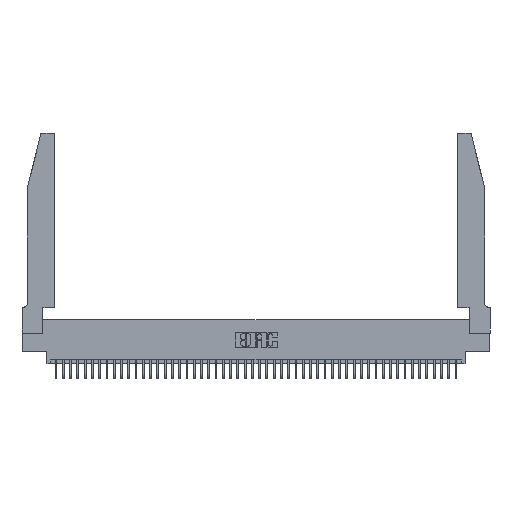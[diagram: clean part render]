
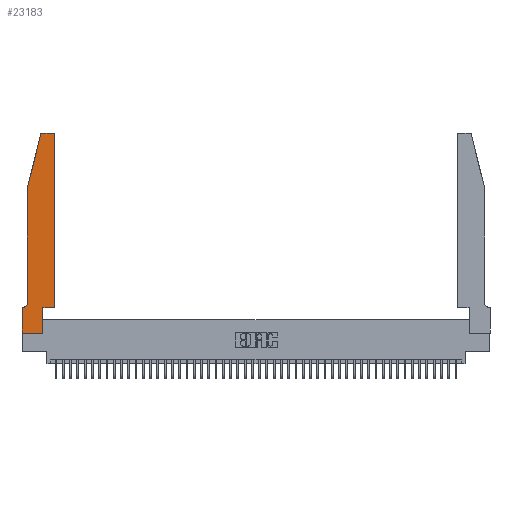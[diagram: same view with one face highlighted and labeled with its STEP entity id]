
A CAD part, top view. The second image highlights one B-rep face of the part: STEP entity #23183.
In plain terms, the highlighted planar face has unit normal (0, 0, 1).
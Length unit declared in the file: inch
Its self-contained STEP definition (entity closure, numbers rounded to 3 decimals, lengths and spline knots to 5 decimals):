
#257 = EDGE_CURVE ( 'NONE', #10455, #32081, #35449, .T. ) ;
#485 = VECTOR ( 'NONE', #39460, 39.37008 ) ;
#1752 = DIRECTION ( 'NONE',  ( 1., 0., 0. ) ) ;
#1906 = ORIENTED_EDGE ( 'NONE', *, *, #47987, .T. ) ;
#2184 = CARTESIAN_POINT ( 'NONE',  ( 0., 0.35, 0.37 ) ) ;
#2358 = DIRECTION ( 'NONE',  ( 1., 0., 0. ) ) ;
#2949 = CARTESIAN_POINT ( 'NONE',  ( 0.284, 2.72, 0.37 ) ) ;
#3360 = LINE ( 'NONE', #16788, #43288 ) ;
#3630 = CARTESIAN_POINT ( 'NONE',  ( 0.4205, 2.72, 0.37 ) ) ;
#4280 = VECTOR ( 'NONE', #7873, 39.37008 ) ;
#4769 = VERTEX_POINT ( 'NONE', #36016 ) ;
#4909 = AXIS2_PLACEMENT_3D ( 'NONE', #2184, #25086, #2358 ) ;
#5660 = CARTESIAN_POINT ( 'NONE',  ( 0.284, 2.75, 0.37 ) ) ;
#5737 = CARTESIAN_POINT ( 'NONE',  ( 0.4505, 0.35, 0.37 ) ) ;
#6211 = ORIENTED_EDGE ( 'NONE', *, *, #22383, .T. ) ;
#6527 = EDGE_CURVE ( 'NONE', #10375, #11061, #22239, .T. ) ;
#6867 = DIRECTION ( 'NONE',  ( 1., 0., 0. ) ) ;
#7563 = DIRECTION ( 'NONE',  ( 1., 0., 0. ) ) ;
#7873 = DIRECTION ( 'NONE',  ( 0., 1., 0. ) ) ;
#10061 = LINE ( 'NONE', #23931, #38669 ) ;
#10171 = LINE ( 'NONE', #46682, #19089 ) ;
#10375 = VERTEX_POINT ( 'NONE', #46897 ) ;
#10455 = VERTEX_POINT ( 'NONE', #28795 ) ;
#10740 = CARTESIAN_POINT ( 'NONE',  ( 0.4505, 0.35, 0.37 ) ) ;
#11061 = VERTEX_POINT ( 'NONE', #5660 ) ;
#11634 = ORIENTED_EDGE ( 'NONE', *, *, #18474, .T. ) ;
#11763 = CARTESIAN_POINT ( 'NONE',  ( 0.0055, 0.35, 0.37 ) ) ;
#12152 = DIRECTION ( 'NONE',  ( 0., 0., -1. ) ) ;
#12297 = ORIENTED_EDGE ( 'NONE', *, *, #15360, .T. ) ;
#14671 = VERTEX_POINT ( 'NONE', #47260 ) ;
#14941 = VERTEX_POINT ( 'NONE', #41276 ) ;
#15360 = EDGE_CURVE ( 'NONE', #37790, #4769, #41450, .T. ) ;
#15671 = VECTOR ( 'NONE', #40970, 39.37008 ) ;
#16411 = AXIS2_PLACEMENT_3D ( 'NONE', #34490, #12152, #38216 ) ;
#16788 = CARTESIAN_POINT ( 'NONE',  ( 0.0755, 2., 0.37 ) ) ;
#17345 = EDGE_CURVE ( 'NONE', #47071, #14671, #29085, .T. ) ;
#17365 = CARTESIAN_POINT ( 'NONE',  ( 0.2605, 2.75, 0.37 ) ) ;
#18474 = EDGE_CURVE ( 'NONE', #14671, #42699, #21819, .T. ) ;
#19089 = VECTOR ( 'NONE', #1752, 39.37008 ) ;
#20352 = CIRCLE ( 'NONE', #20672, 0.03 ) ;
#20645 = VECTOR ( 'NONE', #39708, 39.37008 ) ;
#20672 = AXIS2_PLACEMENT_3D ( 'NONE', #3630, #30081, #7563 ) ;
#21819 = LINE ( 'NONE', #35990, #20645 ) ;
#21844 = EDGE_CURVE ( 'NONE', #26323, #47071, #22605, .T. ) ;
#22239 = LINE ( 'NONE', #17365, #32104 ) ;
#22383 = EDGE_CURVE ( 'NONE', #42699, #10455, #10171, .T. ) ;
#22605 = CIRCLE ( 'NONE', #16411, 0.07 ) ;
#23183 = ADVANCED_FACE ( 'NONE', ( #42199 ), #32407, .T. ) ;
#23386 = ORIENTED_EDGE ( 'NONE', *, *, #31777, .T. ) ;
#23844 = CARTESIAN_POINT ( 'NONE',  ( 0.4505, 0.35, 0.37 ) ) ;
#23931 = CARTESIAN_POINT ( 'NONE',  ( 0.0755, 2., 0.37 ) ) ;
#24482 = ORIENTED_EDGE ( 'NONE', *, *, #30125, .T. ) ;
#25086 = DIRECTION ( 'NONE',  ( 0., 0., 1. ) ) ;
#25728 = ORIENTED_EDGE ( 'NONE', *, *, #27116, .T. ) ;
#25966 = VERTEX_POINT ( 'NONE', #30491 ) ;
#26323 = VERTEX_POINT ( 'NONE', #35918 ) ;
#27116 = EDGE_CURVE ( 'NONE', #4769, #10375, #20352, .T. ) ;
#27422 = ORIENTED_EDGE ( 'NONE', *, *, #43265, .T. ) ;
#27886 = DIRECTION ( 'NONE',  ( -0.239, -0.971, 0. ) ) ;
#28019 = ORIENTED_EDGE ( 'NONE', *, *, #17345, .T. ) ;
#28795 = CARTESIAN_POINT ( 'NONE',  ( 0.2865, 0., 0.37 ) ) ;
#29085 = LINE ( 'NONE', #48417, #15671 ) ;
#29406 = DIRECTION ( 'NONE',  ( 0., 0., 1. ) ) ;
#29792 = ORIENTED_EDGE ( 'NONE', *, *, #257, .T. ) ;
#30081 = DIRECTION ( 'NONE',  ( 0., 0., 1. ) ) ;
#30104 = CARTESIAN_POINT ( 'NONE',  ( 0.2865, 0.35, 0.37 ) ) ;
#30125 = EDGE_CURVE ( 'NONE', #25966, #26323, #10061, .T. ) ;
#30491 = CARTESIAN_POINT ( 'NONE',  ( 0.0755, 2., 0.37 ) ) ;
#30708 = LINE ( 'NONE', #5737, #485 ) ;
#31439 = DIRECTION ( 'NONE',  ( 0., -1., 0. ) ) ;
#31600 = VECTOR ( 'NONE', #40554, 39.37008 ) ;
#31777 = EDGE_CURVE ( 'NONE', #32081, #37790, #30708, .T. ) ;
#32081 = VERTEX_POINT ( 'NONE', #30104 ) ;
#32104 = VECTOR ( 'NONE', #43339, 39.37008 ) ;
#32407 = PLANE ( 'NONE',  #4909 ) ;
#34086 = CARTESIAN_POINT ( 'NONE',  ( 0.2865, 0.35, 0.37 ) ) ;
#34490 = CARTESIAN_POINT ( 'NONE',  ( 0.0055, 0.42, 0.37 ) ) ;
#35360 = AXIS2_PLACEMENT_3D ( 'NONE', #2949, #29406, #6867 ) ;
#35449 = LINE ( 'NONE', #34086, #4280 ) ;
#35918 = CARTESIAN_POINT ( 'NONE',  ( 0.0755, 0.42, 0.37 ) ) ;
#35990 = CARTESIAN_POINT ( 'NONE',  ( 0., 0., 0.37 ) ) ;
#36016 = CARTESIAN_POINT ( 'NONE',  ( 0.4505, 2.72, 0.37 ) ) ;
#36074 = ORIENTED_EDGE ( 'NONE', *, *, #6527, .T. ) ;
#37790 = VERTEX_POINT ( 'NONE', #23844 ) ;
#38216 = DIRECTION ( 'NONE',  ( -1., 0., 0. ) ) ;
#38669 = VECTOR ( 'NONE', #31439, 39.37008 ) ;
#38828 = EDGE_LOOP ( 'NONE', ( #36074, #27422, #1906, #24482, #40158, #28019, #11634, #6211, #29792, #23386, #12297, #25728 ) ) ;
#39460 = DIRECTION ( 'NONE',  ( 1., 0., 0. ) ) ;
#39708 = DIRECTION ( 'NONE',  ( 0., -1., 0. ) ) ;
#40158 = ORIENTED_EDGE ( 'NONE', *, *, #21844, .T. ) ;
#40554 = DIRECTION ( 'NONE',  ( 0., 1., 0. ) ) ;
#40970 = DIRECTION ( 'NONE',  ( -1., 0., 0. ) ) ;
#41276 = CARTESIAN_POINT ( 'NONE',  ( 0.25487, 2.72718, 0.37 ) ) ;
#41450 = LINE ( 'NONE', #10740, #31600 ) ;
#42199 = FACE_OUTER_BOUND ( 'NONE', #38828, .T. ) ;
#42699 = VERTEX_POINT ( 'NONE', #47277 ) ;
#43265 = EDGE_CURVE ( 'NONE', #11061, #14941, #46543, .T. ) ;
#43288 = VECTOR ( 'NONE', #27886, 39.37008 ) ;
#43339 = DIRECTION ( 'NONE',  ( -1., 0., 0. ) ) ;
#46543 = CIRCLE ( 'NONE', #35360, 0.03 ) ;
#46682 = CARTESIAN_POINT ( 'NONE',  ( 0., 0., 0.37 ) ) ;
#46897 = CARTESIAN_POINT ( 'NONE',  ( 0.4205, 2.75, 0.37 ) ) ;
#47071 = VERTEX_POINT ( 'NONE', #11763 ) ;
#47260 = CARTESIAN_POINT ( 'NONE',  ( 0., 0.35, 0.37 ) ) ;
#47277 = CARTESIAN_POINT ( 'NONE',  ( 0., 0., 0.37 ) ) ;
#47987 = EDGE_CURVE ( 'NONE', #14941, #25966, #3360, .T. ) ;
#48417 = CARTESIAN_POINT ( 'NONE',  ( 0.0755, 0.35, 0.37 ) ) ;
